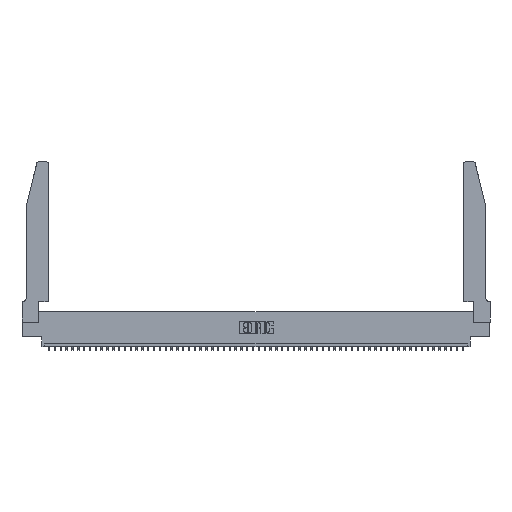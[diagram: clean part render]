
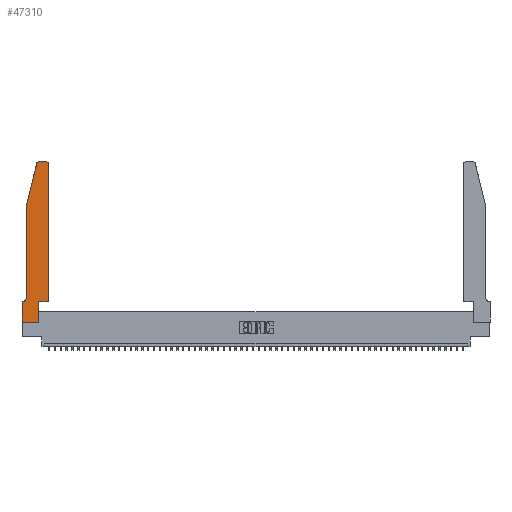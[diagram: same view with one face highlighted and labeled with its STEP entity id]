
A CAD part, top view. The second image highlights one B-rep face of the part: STEP entity #47310.
In plain terms, the highlighted planar face has unit normal (0, 0, 1).
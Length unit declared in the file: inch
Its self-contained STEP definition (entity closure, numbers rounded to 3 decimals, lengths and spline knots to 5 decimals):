
#113 = LINE ( 'NONE', #22895, #48717 ) ;
#1025 = ORIENTED_EDGE ( 'NONE', *, *, #20557, .T. ) ;
#1352 = AXIS2_PLACEMENT_3D ( 'NONE', #16186, #16928, #33734 ) ;
#1798 = VERTEX_POINT ( 'NONE', #4695 ) ;
#2625 = CARTESIAN_POINT ( 'NONE',  ( 0.0755, 0.42, 0.37 ) ) ;
#2767 = DIRECTION ( 'NONE',  ( 1., 0., 0. ) ) ;
#3055 = CARTESIAN_POINT ( 'NONE',  ( 0., 0., 0.37 ) ) ;
#3112 = EDGE_CURVE ( 'NONE', #7821, #48602, #17850, .T. ) ;
#3248 = EDGE_CURVE ( 'NONE', #48602, #1798, #47846, .T. ) ;
#3602 = EDGE_LOOP ( 'NONE', ( #21786, #22652, #52198, #52042, #53513, #34567, #16629, #1025, #54565, #8378, #34426, #6787 ) ) ;
#3943 = AXIS2_PLACEMENT_3D ( 'NONE', #53900, #20001, #15724 ) ;
#4695 = CARTESIAN_POINT ( 'NONE',  ( 0.25487, 2.72718, 0.37 ) ) ;
#5029 = EDGE_CURVE ( 'NONE', #27996, #48088, #27905, .T. ) ;
#6787 = ORIENTED_EDGE ( 'NONE', *, *, #38875, .T. ) ;
#7009 = CARTESIAN_POINT ( 'NONE',  ( 0.284, 2.72, 0.37 ) ) ;
#7821 = VERTEX_POINT ( 'NONE', #52028 ) ;
#8115 = DIRECTION ( 'NONE',  ( 0., 1., 0. ) ) ;
#8378 = ORIENTED_EDGE ( 'NONE', *, *, #5029, .T. ) ;
#9674 = FACE_OUTER_BOUND ( 'NONE', #3602, .T. ) ;
#10025 = CARTESIAN_POINT ( 'NONE',  ( 0., 0., 0.37 ) ) ;
#11906 = DIRECTION ( 'NONE',  ( 0., 0., -1. ) ) ;
#11927 = CARTESIAN_POINT ( 'NONE',  ( 0.0755, 0.35, 0.37 ) ) ;
#12217 = VECTOR ( 'NONE', #8115, 39.37008 ) ;
#14897 = LINE ( 'NONE', #29741, #12217 ) ;
#15724 = DIRECTION ( 'NONE',  ( 1., 0., 0. ) ) ;
#16186 = CARTESIAN_POINT ( 'NONE',  ( 0., 0.35, 0.37 ) ) ;
#16309 = EDGE_CURVE ( 'NONE', #47466, #50610, #48491, .T. ) ;
#16629 = ORIENTED_EDGE ( 'NONE', *, *, #18942, .T. ) ;
#16656 = CARTESIAN_POINT ( 'NONE',  ( 0.0755, 2., 0.37 ) ) ;
#16928 = DIRECTION ( 'NONE',  ( 0., 0., 1. ) ) ;
#16972 = EDGE_CURVE ( 'NONE', #1798, #29653, #35610, .T. ) ;
#17758 = LINE ( 'NONE', #10025, #47751 ) ;
#17850 = LINE ( 'NONE', #35901, #31170 ) ;
#18365 = AXIS2_PLACEMENT_3D ( 'NONE', #7009, #49649, #2767 ) ;
#18942 = EDGE_CURVE ( 'NONE', #50610, #21079, #39365, .T. ) ;
#20001 = DIRECTION ( 'NONE',  ( 0., 0., 1. ) ) ;
#20557 = EDGE_CURVE ( 'NONE', #21079, #21236, #17758, .T. ) ;
#21079 = VERTEX_POINT ( 'NONE', #52067 ) ;
#21236 = VERTEX_POINT ( 'NONE', #27475 ) ;
#21786 = ORIENTED_EDGE ( 'NONE', *, *, #3112, .T. ) ;
#22652 = ORIENTED_EDGE ( 'NONE', *, *, #3248, .T. ) ;
#22724 = VERTEX_POINT ( 'NONE', #2625 ) ;
#22895 = CARTESIAN_POINT ( 'NONE',  ( 0.0755, 2., 0.37 ) ) ;
#23361 = VECTOR ( 'NONE', #30424, 39.37008 ) ;
#25300 = PLANE ( 'NONE',  #1352 ) ;
#27320 = DIRECTION ( 'NONE',  ( 1., 0., 0. ) ) ;
#27475 = CARTESIAN_POINT ( 'NONE',  ( 0.2865, 0., 0.37 ) ) ;
#27905 = LINE ( 'NONE', #36083, #53210 ) ;
#27996 = VERTEX_POINT ( 'NONE', #31304 ) ;
#29301 = CARTESIAN_POINT ( 'NONE',  ( 0.284, 2.75, 0.37 ) ) ;
#29405 = CIRCLE ( 'NONE', #3943, 0.03 ) ;
#29441 = DIRECTION ( 'NONE',  ( -1., 0., 0. ) ) ;
#29653 = VERTEX_POINT ( 'NONE', #16656 ) ;
#29741 = CARTESIAN_POINT ( 'NONE',  ( 0.4505, 0.35, 0.37 ) ) ;
#30424 = DIRECTION ( 'NONE',  ( 0., 1., 0. ) ) ;
#31170 = VECTOR ( 'NONE', #52456, 39.37008 ) ;
#31304 = CARTESIAN_POINT ( 'NONE',  ( 0.2865, 0.35, 0.37 ) ) ;
#31986 = VECTOR ( 'NONE', #50304, 39.37008 ) ;
#32041 = LINE ( 'NONE', #43088, #23361 ) ;
#32140 = EDGE_CURVE ( 'NONE', #29653, #22724, #113, .T. ) ;
#33734 = DIRECTION ( 'NONE',  ( 1., 0., 0. ) ) ;
#34057 = DIRECTION ( 'NONE',  ( -0.239, -0.971, 0. ) ) ;
#34209 = CARTESIAN_POINT ( 'NONE',  ( 0.4505, 0.35, 0.37 ) ) ;
#34426 = ORIENTED_EDGE ( 'NONE', *, *, #37657, .T. ) ;
#34567 = ORIENTED_EDGE ( 'NONE', *, *, #16309, .T. ) ;
#35167 = EDGE_CURVE ( 'NONE', #22724, #47466, #35692, .T. ) ;
#35610 = LINE ( 'NONE', #37952, #52375 ) ;
#35692 = CIRCLE ( 'NONE', #38757, 0.07 ) ;
#35901 = CARTESIAN_POINT ( 'NONE',  ( 0.2605, 2.75, 0.37 ) ) ;
#36083 = CARTESIAN_POINT ( 'NONE',  ( 0.4505, 0.35, 0.37 ) ) ;
#37657 = EDGE_CURVE ( 'NONE', #48088, #43134, #14897, .T. ) ;
#37952 = CARTESIAN_POINT ( 'NONE',  ( 0.0755, 2., 0.37 ) ) ;
#38757 = AXIS2_PLACEMENT_3D ( 'NONE', #45641, #11906, #45284 ) ;
#38875 = EDGE_CURVE ( 'NONE', #43134, #7821, #29405, .T. ) ;
#39131 = DIRECTION ( 'NONE',  ( 1., 0., 0. ) ) ;
#39365 = LINE ( 'NONE', #3055, #31986 ) ;
#40225 = DIRECTION ( 'NONE',  ( 0., -1., 0. ) ) ;
#42993 = CARTESIAN_POINT ( 'NONE',  ( 0., 0.35, 0.37 ) ) ;
#43088 = CARTESIAN_POINT ( 'NONE',  ( 0.2865, 0.35, 0.37 ) ) ;
#43134 = VERTEX_POINT ( 'NONE', #50418 ) ;
#45284 = DIRECTION ( 'NONE',  ( -1., 0., 0. ) ) ;
#45641 = CARTESIAN_POINT ( 'NONE',  ( 0.0055, 0.42, 0.37 ) ) ;
#47305 = CARTESIAN_POINT ( 'NONE',  ( 0.0055, 0.35, 0.37 ) ) ;
#47310 = ADVANCED_FACE ( 'NONE', ( #9674 ), #25300, .T. ) ;
#47466 = VERTEX_POINT ( 'NONE', #47305 ) ;
#47751 = VECTOR ( 'NONE', #39131, 39.37008 ) ;
#47846 = CIRCLE ( 'NONE', #18365, 0.03 ) ;
#48088 = VERTEX_POINT ( 'NONE', #34209 ) ;
#48491 = LINE ( 'NONE', #11927, #53803 ) ;
#48602 = VERTEX_POINT ( 'NONE', #29301 ) ;
#48717 = VECTOR ( 'NONE', #40225, 39.37008 ) ;
#49649 = DIRECTION ( 'NONE',  ( 0., 0., 1. ) ) ;
#50304 = DIRECTION ( 'NONE',  ( 0., -1., 0. ) ) ;
#50418 = CARTESIAN_POINT ( 'NONE',  ( 0.4505, 2.72, 0.37 ) ) ;
#50610 = VERTEX_POINT ( 'NONE', #42993 ) ;
#52028 = CARTESIAN_POINT ( 'NONE',  ( 0.4205, 2.75, 0.37 ) ) ;
#52042 = ORIENTED_EDGE ( 'NONE', *, *, #32140, .T. ) ;
#52067 = CARTESIAN_POINT ( 'NONE',  ( 0., 0., 0.37 ) ) ;
#52198 = ORIENTED_EDGE ( 'NONE', *, *, #16972, .T. ) ;
#52375 = VECTOR ( 'NONE', #34057, 39.37008 ) ;
#52456 = DIRECTION ( 'NONE',  ( -1., 0., 0. ) ) ;
#53210 = VECTOR ( 'NONE', #27320, 39.37008 ) ;
#53513 = ORIENTED_EDGE ( 'NONE', *, *, #35167, .T. ) ;
#53803 = VECTOR ( 'NONE', #29441, 39.37008 ) ;
#53900 = CARTESIAN_POINT ( 'NONE',  ( 0.4205, 2.72, 0.37 ) ) ;
#54565 = ORIENTED_EDGE ( 'NONE', *, *, #54948, .T. ) ;
#54948 = EDGE_CURVE ( 'NONE', #21236, #27996, #32041, .T. ) ;
